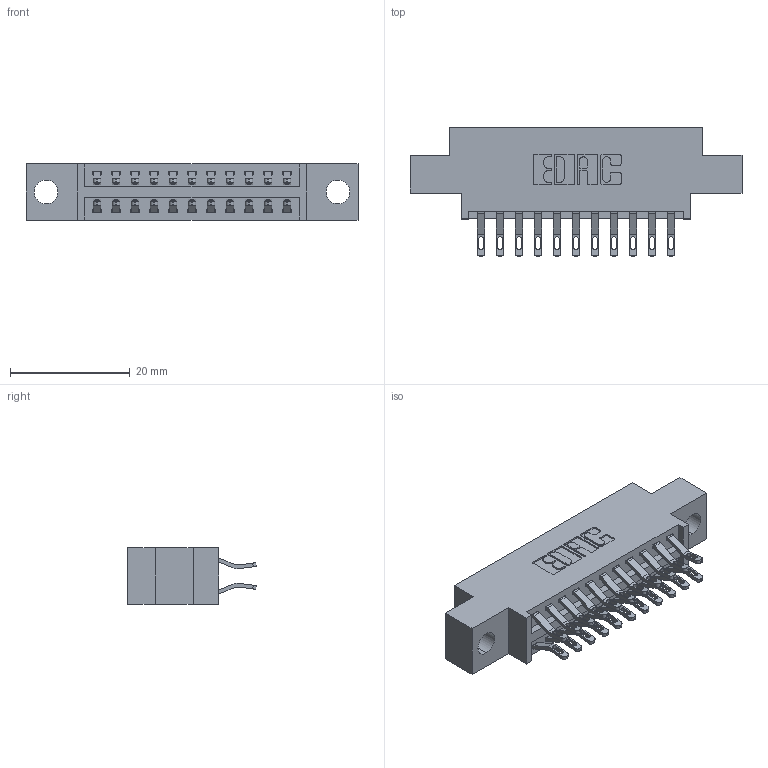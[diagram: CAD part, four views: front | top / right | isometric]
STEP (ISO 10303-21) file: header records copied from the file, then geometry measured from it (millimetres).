
FILE_DESCRIPTION (( 'STEP AP203' ), '1' );
FILE_NAME ('346-022-555-804.STEP', '2022-05-18T21:43:29', ( '' ), ( '' ), 'SwSTEP 2.0', 'SolidWorks 2020', '' );
FILE_SCHEMA (( 'CONFIG_CONTROL_DESIGN' ));
Length unit declared in the file: inch
Products named in the file (3): 345-292-001_555 Tail; 346 Part_0.170 Offset - 0.156 Dia-TH; 346-022-555-804
Assembly tree (23 placements, depth 2):
  346-022-555-804
    346 Part_0.170 Offset - 0.156 Dia-TH
    345-292-001_555 Tail  x22
Bounding box: 55.5 x 21.46 x 9.4 mm (x, y, z)
Volume: 4974.3 mm3; surface area: 6605.3 mm2
Topology: 23 solids, 23 shells, 1416 faces, 4403 edges, 2934 vertices
Faces by surface type: plane 820, cylinder 596
Entity records: 12229 total; most frequent: CARTESIAN_POINT 2100, ORIENTED_EDGE 2002, DIRECTION 1869, EDGE_CURVE 1001, VECTOR 805, LINE 805, VERTEX_POINT 666, AXIS2_PLACEMENT_3D 532
